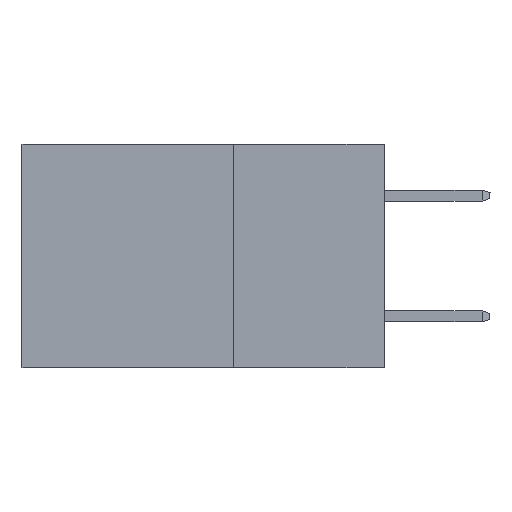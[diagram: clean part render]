
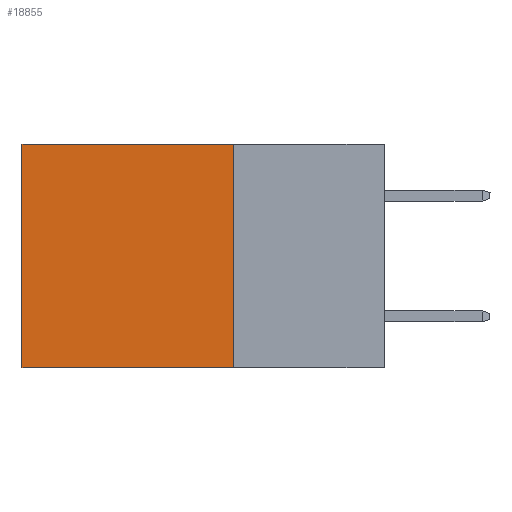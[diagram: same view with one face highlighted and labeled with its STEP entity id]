
A CAD part, left-side view. The second image highlights one B-rep face of the part: STEP entity #18855.
In plain terms, the highlighted planar face has unit normal (-1, 0, 0).
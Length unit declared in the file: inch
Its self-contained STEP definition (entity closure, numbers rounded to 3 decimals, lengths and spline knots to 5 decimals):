
#25 = ORIENTED_EDGE ( 'NONE', *, *, #5132, .T. ) ;
#3154 = ORIENTED_EDGE ( 'NONE', *, *, #18263, .F. ) ;
#3559 = LINE ( 'NONE', #24637, #16985 ) ;
#5132 = EDGE_CURVE ( 'NONE', #29604, #12373, #3559, .T. ) ;
#5594 = VECTOR ( 'NONE', #19375, 39.37008 ) ;
#7491 = DIRECTION ( 'NONE',  ( 0., 0., -1. ) ) ;
#7735 = EDGE_CURVE ( 'NONE', #29604, #14234, #19936, .T. ) ;
#9291 = PLANE ( 'NONE',  #13666 ) ;
#9821 = LINE ( 'NONE', #26753, #5594 ) ;
#10461 = CARTESIAN_POINT ( 'NONE',  ( 0.298, 0.25, 0. ) ) ;
#10581 = FACE_OUTER_BOUND ( 'NONE', #11195, .T. ) ;
#11195 = EDGE_LOOP ( 'NONE', ( #18976, #3154, #24760, #25 ) ) ;
#12373 = VERTEX_POINT ( 'NONE', #18359 ) ;
#13666 = AXIS2_PLACEMENT_3D ( 'NONE', #26604, #31670, #19332 ) ;
#14234 = VERTEX_POINT ( 'NONE', #14640 ) ;
#14640 = CARTESIAN_POINT ( 'NONE',  ( 0.298, 0.25, -0.37 ) ) ;
#15236 = DIRECTION ( 'NONE',  ( 0., 1., 0. ) ) ;
#15703 = VECTOR ( 'NONE', #25594, 39.37008 ) ;
#16985 = VECTOR ( 'NONE', #15236, 39.37008 ) ;
#18263 = EDGE_CURVE ( 'NONE', #14234, #29280, #9821, .T. ) ;
#18359 = CARTESIAN_POINT ( 'NONE',  ( 0.298, 0.6, 0. ) ) ;
#18855 = ADVANCED_FACE ( 'NONE', ( #10581 ), #9291, .F. ) ;
#18976 = ORIENTED_EDGE ( 'NONE', *, *, #25492, .T. ) ;
#19332 = DIRECTION ( 'NONE',  ( 0., 0., -1. ) ) ;
#19375 = DIRECTION ( 'NONE',  ( 0., 1., 0. ) ) ;
#19936 = LINE ( 'NONE', #10461, #15703 ) ;
#21814 = VECTOR ( 'NONE', #7491, 39.37008 ) ;
#22501 = CARTESIAN_POINT ( 'NONE',  ( 0.298, 0.6, 0. ) ) ;
#24163 = CARTESIAN_POINT ( 'NONE',  ( 0.298, 0.6, -0.37 ) ) ;
#24637 = CARTESIAN_POINT ( 'NONE',  ( 0.298, 0.25, 0. ) ) ;
#24760 = ORIENTED_EDGE ( 'NONE', *, *, #7735, .F. ) ;
#24880 = CARTESIAN_POINT ( 'NONE',  ( 0.298, 0.25, 0. ) ) ;
#25492 = EDGE_CURVE ( 'NONE', #12373, #29280, #28414, .T. ) ;
#25594 = DIRECTION ( 'NONE',  ( 0., 0., -1. ) ) ;
#26604 = CARTESIAN_POINT ( 'NONE',  ( 0.298, 0.25, 0. ) ) ;
#26753 = CARTESIAN_POINT ( 'NONE',  ( 0.298, 0.25, -0.37 ) ) ;
#28414 = LINE ( 'NONE', #22501, #21814 ) ;
#29280 = VERTEX_POINT ( 'NONE', #24163 ) ;
#29604 = VERTEX_POINT ( 'NONE', #24880 ) ;
#31670 = DIRECTION ( 'NONE',  ( 1., 0., 0. ) ) ;
